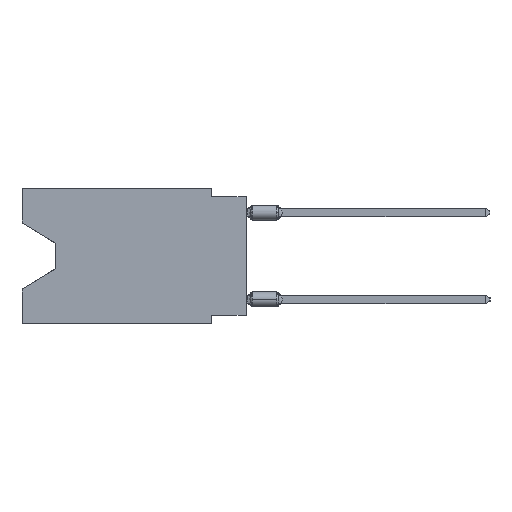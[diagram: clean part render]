
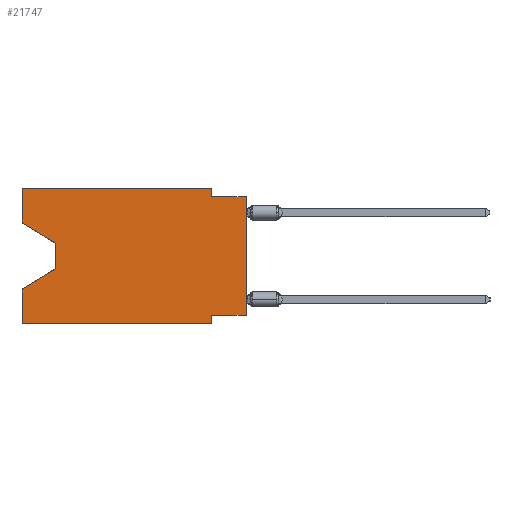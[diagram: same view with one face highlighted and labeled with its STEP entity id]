
A CAD part, left-side view. The second image highlights one B-rep face of the part: STEP entity #21747.
In plain terms, the highlighted planar face has unit normal (-1, 0, 0).
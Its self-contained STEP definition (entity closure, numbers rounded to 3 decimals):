
#882 = LINE ( 'NONE', #9396, #4574 ) ;
#921 = CARTESIAN_POINT ( 'NONE',  ( 0., 13.97, -5.893 ) ) ;
#1022 = EDGE_CURVE ( 'NONE', #4767, #26354, #2007, .T. ) ;
#1617 = VECTOR ( 'NONE', #14435, 1000. ) ;
#1933 = VERTEX_POINT ( 'NONE', #11959 ) ;
#2007 = LINE ( 'NONE', #34104, #10886 ) ;
#2265 = VERTEX_POINT ( 'NONE', #28109 ) ;
#3470 = DIRECTION ( 'NONE',  ( 0., -1., 0. ) ) ;
#3739 = PLANE ( 'NONE',  #7528 ) ;
#4574 = VECTOR ( 'NONE', #18088, 1000. ) ;
#4767 = VERTEX_POINT ( 'NONE', #5707 ) ;
#4814 = ORIENTED_EDGE ( 'NONE', *, *, #26882, .F. ) ;
#5462 = ORIENTED_EDGE ( 'NONE', *, *, #14211, .F. ) ;
#5680 = ORIENTED_EDGE ( 'NONE', *, *, #32586, .T. ) ;
#5707 = CARTESIAN_POINT ( 'NONE',  ( 0., 2.54, 0. ) ) ;
#6328 = ORIENTED_EDGE ( 'NONE', *, *, #36284, .T. ) ;
#6386 = CARTESIAN_POINT ( 'NONE',  ( 0., 16.383, 0. ) ) ;
#6857 = EDGE_CURVE ( 'NONE', #13538, #2265, #33497, .T. ) ;
#7036 = DIRECTION ( 'NONE',  ( 0., 0., 1. ) ) ;
#7528 = AXIS2_PLACEMENT_3D ( 'NONE', #27328, #10106, #21897 ) ;
#7662 = VECTOR ( 'NONE', #18160, 1000. ) ;
#8336 = VECTOR ( 'NONE', #16952, 1000. ) ;
#8519 = ORIENTED_EDGE ( 'NONE', *, *, #14551, .F. ) ;
#9131 = VERTEX_POINT ( 'NONE', #12191 ) ;
#9249 = LINE ( 'NONE', #921, #23874 ) ;
#9396 = CARTESIAN_POINT ( 'NONE',  ( 0., 13.97, -4.013 ) ) ;
#9849 = CARTESIAN_POINT ( 'NONE',  ( 0., 16.383, -9.906 ) ) ;
#9925 = FACE_OUTER_BOUND ( 'NONE', #28586, .T. ) ;
#10106 = DIRECTION ( 'NONE',  ( 1., 0., 0. ) ) ;
#10403 = CARTESIAN_POINT ( 'NONE',  ( 0., 16.383, 0. ) ) ;
#10500 = LINE ( 'NONE', #24625, #20762 ) ;
#10849 = VECTOR ( 'NONE', #3470, 1000. ) ;
#10886 = VECTOR ( 'NONE', #22715, 1000. ) ;
#11388 = CARTESIAN_POINT ( 'NONE',  ( 0., 2.54, -9.271 ) ) ;
#11959 = CARTESIAN_POINT ( 'NONE',  ( 0., 0., -0.635 ) ) ;
#12121 = CARTESIAN_POINT ( 'NONE',  ( 0., 0., -9.271 ) ) ;
#12191 = CARTESIAN_POINT ( 'NONE',  ( 0., 16.383, -2.546 ) ) ;
#12295 = LINE ( 'NONE', #24258, #24985 ) ;
#13538 = VERTEX_POINT ( 'NONE', #13667 ) ;
#13667 = CARTESIAN_POINT ( 'NONE',  ( 0., 16.383, -9.906 ) ) ;
#14211 = EDGE_CURVE ( 'NONE', #23883, #4767, #31046, .T. ) ;
#14435 = DIRECTION ( 'NONE',  ( 0., 0., -1. ) ) ;
#14551 = EDGE_CURVE ( 'NONE', #28442, #31041, #18092, .T. ) ;
#14641 = LINE ( 'NONE', #37640, #1617 ) ;
#14733 = CARTESIAN_POINT ( 'NONE',  ( 0., 13.97, -5.893 ) ) ;
#15081 = EDGE_CURVE ( 'NONE', #9131, #36634, #10500, .T. ) ;
#15173 = DIRECTION ( 'NONE',  ( 0., -1., 0. ) ) ;
#16952 = DIRECTION ( 'NONE',  ( 0., 0., 1. ) ) ;
#17222 = VERTEX_POINT ( 'NONE', #14733 ) ;
#18088 = DIRECTION ( 'NONE',  ( 0., 0., -1. ) ) ;
#18092 = LINE ( 'NONE', #12121, #25640 ) ;
#18160 = DIRECTION ( 'NONE',  ( 0., 0., 1. ) ) ;
#18683 = DIRECTION ( 'NONE',  ( 0., 0.855, -0.519 ) ) ;
#18804 = ORIENTED_EDGE ( 'NONE', *, *, #1022, .F. ) ;
#20762 = VECTOR ( 'NONE', #27893, 1000. ) ;
#21747 = ADVANCED_FACE ( 'NONE', ( #9925 ), #3739, .F. ) ;
#21829 = CARTESIAN_POINT ( 'NONE',  ( 0., 16.383, 0. ) ) ;
#21897 = DIRECTION ( 'NONE',  ( 0., 0., -1. ) ) ;
#22715 = DIRECTION ( 'NONE',  ( 0., 0., -1. ) ) ;
#22724 = ORIENTED_EDGE ( 'NONE', *, *, #34767, .F. ) ;
#23874 = VECTOR ( 'NONE', #18683, 1000. ) ;
#23883 = VERTEX_POINT ( 'NONE', #21829 ) ;
#24258 = CARTESIAN_POINT ( 'NONE',  ( 0., 0., -0.635 ) ) ;
#24625 = CARTESIAN_POINT ( 'NONE',  ( 0., 16.383, -2.546 ) ) ;
#24985 = VECTOR ( 'NONE', #15173, 1000. ) ;
#25536 = ORIENTED_EDGE ( 'NONE', *, *, #15081, .T. ) ;
#25631 = ORIENTED_EDGE ( 'NONE', *, *, #36576, .F. ) ;
#25640 = VECTOR ( 'NONE', #33168, 1000. ) ;
#26354 = VERTEX_POINT ( 'NONE', #35511 ) ;
#26872 = CARTESIAN_POINT ( 'NONE',  ( 0., 2.54, -9.906 ) ) ;
#26875 = LINE ( 'NONE', #6386, #7662 ) ;
#26882 = EDGE_CURVE ( 'NONE', #26354, #1933, #12295, .T. ) ;
#27328 = CARTESIAN_POINT ( 'NONE',  ( 0., 16.383, 0. ) ) ;
#27873 = EDGE_CURVE ( 'NONE', #17222, #2265, #9249, .T. ) ;
#27893 = DIRECTION ( 'NONE',  ( 0., -0.855, -0.519 ) ) ;
#28109 = CARTESIAN_POINT ( 'NONE',  ( 0., 16.383, -7.36 ) ) ;
#28442 = VERTEX_POINT ( 'NONE', #31704 ) ;
#28586 = EDGE_LOOP ( 'NONE', ( #25536, #37985, #33903, #30234, #6328, #25631, #8519, #5680, #4814, #18804, #5462, #22724 ) ) ;
#29136 = CARTESIAN_POINT ( 'NONE',  ( 0., 13.97, -4.013 ) ) ;
#29949 = EDGE_CURVE ( 'NONE', #36634, #17222, #882, .T. ) ;
#30234 = ORIENTED_EDGE ( 'NONE', *, *, #6857, .F. ) ;
#30498 = LINE ( 'NONE', #9849, #10849 ) ;
#30799 = CARTESIAN_POINT ( 'NONE',  ( 0., 16.383, 0. ) ) ;
#31041 = VERTEX_POINT ( 'NONE', #11388 ) ;
#31046 = LINE ( 'NONE', #10403, #36753 ) ;
#31436 = DIRECTION ( 'NONE',  ( 0., -1., 0. ) ) ;
#31627 = LINE ( 'NONE', #37636, #8336 ) ;
#31704 = CARTESIAN_POINT ( 'NONE',  ( 0., 0., -9.271 ) ) ;
#32319 = VECTOR ( 'NONE', #7036, 1000. ) ;
#32586 = EDGE_CURVE ( 'NONE', #28442, #1933, #31627, .T. ) ;
#33168 = DIRECTION ( 'NONE',  ( 0., 1., 0. ) ) ;
#33497 = LINE ( 'NONE', #30799, #32319 ) ;
#33903 = ORIENTED_EDGE ( 'NONE', *, *, #27873, .T. ) ;
#34104 = CARTESIAN_POINT ( 'NONE',  ( 0., 2.54, 0. ) ) ;
#34767 = EDGE_CURVE ( 'NONE', #9131, #23883, #26875, .T. ) ;
#35511 = CARTESIAN_POINT ( 'NONE',  ( 0., 2.54, -0.635 ) ) ;
#36284 = EDGE_CURVE ( 'NONE', #13538, #37444, #30498, .T. ) ;
#36576 = EDGE_CURVE ( 'NONE', #31041, #37444, #14641, .T. ) ;
#36634 = VERTEX_POINT ( 'NONE', #29136 ) ;
#36753 = VECTOR ( 'NONE', #31436, 1000. ) ;
#37444 = VERTEX_POINT ( 'NONE', #26872 ) ;
#37636 = CARTESIAN_POINT ( 'NONE',  ( 0., 0., 0. ) ) ;
#37640 = CARTESIAN_POINT ( 'NONE',  ( 0., 2.54, -9.906 ) ) ;
#37985 = ORIENTED_EDGE ( 'NONE', *, *, #29949, .T. ) ;
